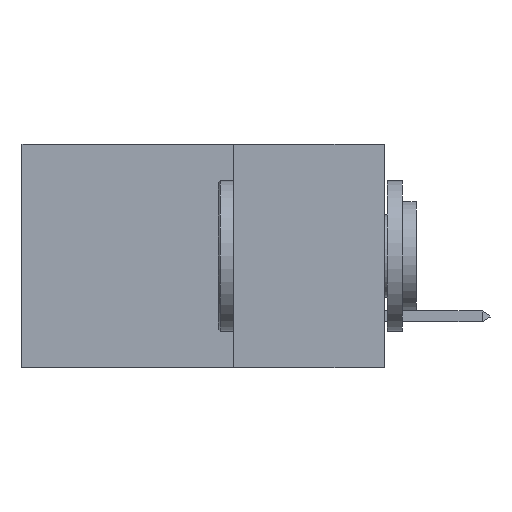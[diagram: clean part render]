
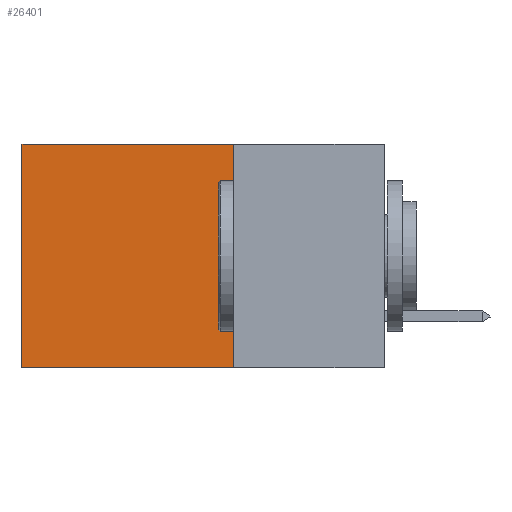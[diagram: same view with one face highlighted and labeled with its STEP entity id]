
A CAD part, left-side view. The second image highlights one B-rep face of the part: STEP entity #26401.
In plain terms, the highlighted planar face has unit normal (-1, 0, 0).
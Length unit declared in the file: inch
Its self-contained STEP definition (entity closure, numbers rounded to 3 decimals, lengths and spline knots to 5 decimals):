
#194 = DIRECTION ( 'NONE',  ( 1., 0., 0. ) ) ;
#1135 = FACE_OUTER_BOUND ( 'NONE', #11363, .T. ) ;
#2732 = LINE ( 'NONE', #25887, #25509 ) ;
#4057 = VECTOR ( 'NONE', #27103, 39.37008 ) ;
#4391 = CARTESIAN_POINT ( 'NONE',  ( 0.2875, 0.6, 0. ) ) ;
#5438 = CARTESIAN_POINT ( 'NONE',  ( 0.2875, 0.6, 0. ) ) ;
#7429 = VECTOR ( 'NONE', #18797, 39.37008 ) ;
#7836 = CARTESIAN_POINT ( 'NONE',  ( 0.2875, 0.25, -0.37 ) ) ;
#8145 = AXIS2_PLACEMENT_3D ( 'NONE', #13929, #194, #19230 ) ;
#9636 = CARTESIAN_POINT ( 'NONE',  ( 0.2875, 0.25, 0. ) ) ;
#9705 = DIRECTION ( 'NONE',  ( 0., 0., -1. ) ) ;
#9823 = ORIENTED_EDGE ( 'NONE', *, *, #23807, .T. ) ;
#10346 = LINE ( 'NONE', #29434, #7429 ) ;
#11093 = PLANE ( 'NONE',  #8145 ) ;
#11363 = EDGE_LOOP ( 'NONE', ( #14256, #22978, #14274, #9823 ) ) ;
#13929 = CARTESIAN_POINT ( 'NONE',  ( 0.2875, 0.25, 0. ) ) ;
#14256 = ORIENTED_EDGE ( 'NONE', *, *, #34300, .T. ) ;
#14274 = ORIENTED_EDGE ( 'NONE', *, *, #28247, .F. ) ;
#16064 = CARTESIAN_POINT ( 'NONE',  ( 0.2875, 0.6, -0.37 ) ) ;
#18797 = DIRECTION ( 'NONE',  ( 0., 1., 0. ) ) ;
#19230 = DIRECTION ( 'NONE',  ( 0., 0., -1. ) ) ;
#21718 = VECTOR ( 'NONE', #22502, 39.37008 ) ;
#22502 = DIRECTION ( 'NONE',  ( 0., 1., 0. ) ) ;
#22978 = ORIENTED_EDGE ( 'NONE', *, *, #27337, .F. ) ;
#23155 = VERTEX_POINT ( 'NONE', #16064 ) ;
#23486 = CARTESIAN_POINT ( 'NONE',  ( 0.2875, 0.25, -0.37 ) ) ;
#23807 = EDGE_CURVE ( 'NONE', #25809, #29424, #10346, .T. ) ;
#25509 = VECTOR ( 'NONE', #9705, 39.37008 ) ;
#25809 = VERTEX_POINT ( 'NONE', #9636 ) ;
#25887 = CARTESIAN_POINT ( 'NONE',  ( 0.2875, 0.25, 0. ) ) ;
#26401 = ADVANCED_FACE ( 'NONE', ( #1135 ), #11093, .F. ) ;
#27103 = DIRECTION ( 'NONE',  ( 0., 0., -1. ) ) ;
#27337 = EDGE_CURVE ( 'NONE', #28261, #23155, #33107, .T. ) ;
#28247 = EDGE_CURVE ( 'NONE', #25809, #28261, #2732, .T. ) ;
#28261 = VERTEX_POINT ( 'NONE', #7836 ) ;
#29424 = VERTEX_POINT ( 'NONE', #4391 ) ;
#29434 = CARTESIAN_POINT ( 'NONE',  ( 0.2875, 0.25, 0. ) ) ;
#32636 = LINE ( 'NONE', #5438, #4057 ) ;
#33107 = LINE ( 'NONE', #23486, #21718 ) ;
#34300 = EDGE_CURVE ( 'NONE', #29424, #23155, #32636, .T. ) ;
